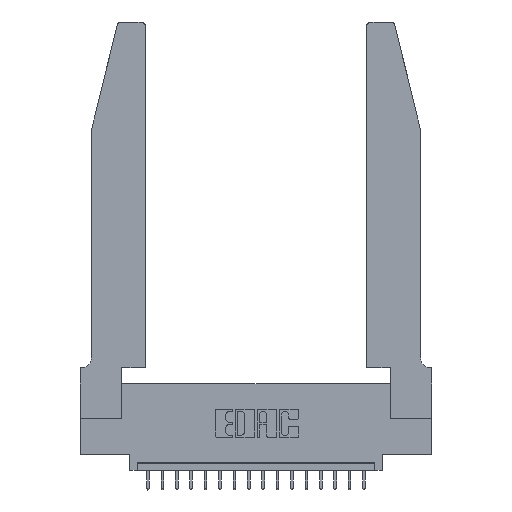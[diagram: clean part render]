
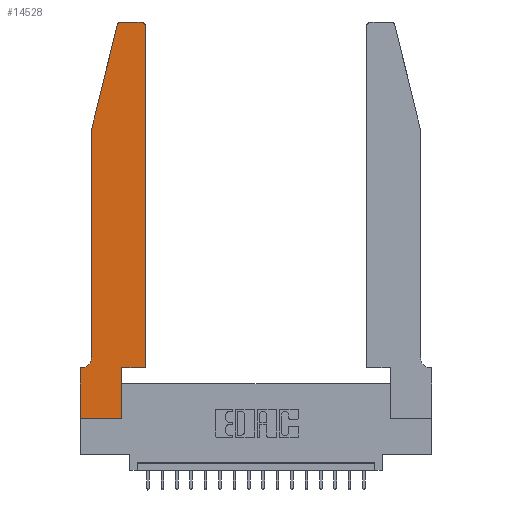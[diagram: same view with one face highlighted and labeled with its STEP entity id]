
A CAD part, top view. The second image highlights one B-rep face of the part: STEP entity #14528.
In plain terms, the highlighted planar face has unit normal (0, 0, 1).
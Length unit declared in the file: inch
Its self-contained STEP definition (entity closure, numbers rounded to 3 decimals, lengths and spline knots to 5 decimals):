
#113 = EDGE_CURVE ( 'NONE', #17525, #18506, #5357, .T. ) ;
#383 = ORIENTED_EDGE ( 'NONE', *, *, #16500, .T. ) ;
#471 = EDGE_CURVE ( 'NONE', #15556, #16411, #1526, .T. ) ;
#630 = EDGE_CURVE ( 'NONE', #4842, #12230, #3383, .T. ) ;
#657 = DIRECTION ( 'NONE',  ( -1., 0., 0. ) ) ;
#890 = DIRECTION ( 'NONE',  ( 0., 0., 1. ) ) ;
#1232 = EDGE_CURVE ( 'NONE', #18089, #17525, #7980, .T. ) ;
#1477 = CARTESIAN_POINT ( 'NONE',  ( 0.284, 2.72, 0.37 ) ) ;
#1526 = LINE ( 'NONE', #9771, #6696 ) ;
#1715 = VECTOR ( 'NONE', #12701, 39.37008 ) ;
#1752 = ORIENTED_EDGE ( 'NONE', *, *, #630, .T. ) ;
#1759 = DIRECTION ( 'NONE',  ( 0., 1., 0. ) ) ;
#1948 = EDGE_CURVE ( 'NONE', #8336, #18089, #7968, .T. ) ;
#2244 = CARTESIAN_POINT ( 'NONE',  ( 0.2865, 0., 0.37 ) ) ;
#2387 = AXIS2_PLACEMENT_3D ( 'NONE', #1477, #890, #7243 ) ;
#2462 = DIRECTION ( 'NONE',  ( 0., -1., 0. ) ) ;
#3156 = VECTOR ( 'NONE', #1759, 39.37008 ) ;
#3383 = CIRCLE ( 'NONE', #2387, 0.03 ) ;
#3620 = ORIENTED_EDGE ( 'NONE', *, *, #471, .T. ) ;
#4023 = VECTOR ( 'NONE', #15811, 39.37008 ) ;
#4216 = ORIENTED_EDGE ( 'NONE', *, *, #17614, .T. ) ;
#4362 = AXIS2_PLACEMENT_3D ( 'NONE', #16031, #18714, #12699 ) ;
#4404 = VERTEX_POINT ( 'NONE', #19523 ) ;
#4630 = DIRECTION ( 'NONE',  ( 1., 0., 0. ) ) ;
#4668 = VECTOR ( 'NONE', #13830, 39.37008 ) ;
#4842 = VERTEX_POINT ( 'NONE', #19663 ) ;
#5047 = CARTESIAN_POINT ( 'NONE',  ( 0.4505, 0.35, 0.37 ) ) ;
#5124 = ORIENTED_EDGE ( 'NONE', *, *, #12304, .T. ) ;
#5357 = CIRCLE ( 'NONE', #4362, 0.03 ) ;
#5645 = ORIENTED_EDGE ( 'NONE', *, *, #17167, .T. ) ;
#5664 = ORIENTED_EDGE ( 'NONE', *, *, #1948, .T. ) ;
#5848 = PLANE ( 'NONE',  #6405 ) ;
#5868 = VERTEX_POINT ( 'NONE', #11637 ) ;
#6051 = CARTESIAN_POINT ( 'NONE',  ( 0.2865, 0.35, 0.37 ) ) ;
#6405 = AXIS2_PLACEMENT_3D ( 'NONE', #20136, #18685, #14142 ) ;
#6568 = DIRECTION ( 'NONE',  ( 0., -1., 0. ) ) ;
#6611 = DIRECTION ( 'NONE',  ( 1., 0., 0. ) ) ;
#6625 = ORIENTED_EDGE ( 'NONE', *, *, #13365, .T. ) ;
#6696 = VECTOR ( 'NONE', #6611, 39.37008 ) ;
#7243 = DIRECTION ( 'NONE',  ( 1., 0., 0. ) ) ;
#7299 = CARTESIAN_POINT ( 'NONE',  ( 0.2605, 2.75, 0.37 ) ) ;
#7926 = CARTESIAN_POINT ( 'NONE',  ( 0.0755, 0.35, 0.37 ) ) ;
#7968 = LINE ( 'NONE', #5047, #11143 ) ;
#7980 = LINE ( 'NONE', #16082, #12696 ) ;
#8004 = CIRCLE ( 'NONE', #11662, 0.07 ) ;
#8146 = LINE ( 'NONE', #19122, #20392 ) ;
#8336 = VERTEX_POINT ( 'NONE', #11892 ) ;
#8852 = VERTEX_POINT ( 'NONE', #17236 ) ;
#9474 = DIRECTION ( 'NONE',  ( 0., 1., 0. ) ) ;
#9771 = CARTESIAN_POINT ( 'NONE',  ( 0., 0., 0.37 ) ) ;
#9949 = EDGE_LOOP ( 'NONE', ( #17696, #1752, #13838, #5645, #5124, #6625, #383, #3620, #4216, #5664, #13246, #10521 ) ) ;
#10457 = LINE ( 'NONE', #7299, #4668 ) ;
#10463 = CARTESIAN_POINT ( 'NONE',  ( 0.4505, 2.72, 0.37 ) ) ;
#10521 = ORIENTED_EDGE ( 'NONE', *, *, #113, .T. ) ;
#11110 = CARTESIAN_POINT ( 'NONE',  ( 0.4505, 0.35, 0.37 ) ) ;
#11143 = VECTOR ( 'NONE', #4630, 39.37008 ) ;
#11169 = EDGE_CURVE ( 'NONE', #18506, #4842, #10457, .T. ) ;
#11637 = CARTESIAN_POINT ( 'NONE',  ( 0.0755, 2., 0.37 ) ) ;
#11662 = AXIS2_PLACEMENT_3D ( 'NONE', #18020, #19658, #657 ) ;
#11877 = CARTESIAN_POINT ( 'NONE',  ( 0.4205, 2.75, 0.37 ) ) ;
#11892 = CARTESIAN_POINT ( 'NONE',  ( 0.2865, 0.35, 0.37 ) ) ;
#12230 = VERTEX_POINT ( 'NONE', #16652 ) ;
#12304 = EDGE_CURVE ( 'NONE', #16963, #4404, #8004, .T. ) ;
#12696 = VECTOR ( 'NONE', #9474, 39.37008 ) ;
#12699 = DIRECTION ( 'NONE',  ( 1., 0., 0. ) ) ;
#12701 = DIRECTION ( 'NONE',  ( -1., 0., 0. ) ) ;
#13188 = LINE ( 'NONE', #7926, #1715 ) ;
#13219 = EDGE_CURVE ( 'NONE', #12230, #5868, #17660, .T. ) ;
#13246 = ORIENTED_EDGE ( 'NONE', *, *, #1232, .T. ) ;
#13361 = CARTESIAN_POINT ( 'NONE',  ( 0.0755, 0.42, 0.37 ) ) ;
#13365 = EDGE_CURVE ( 'NONE', #4404, #8852, #13188, .T. ) ;
#13830 = DIRECTION ( 'NONE',  ( -1., 0., 0. ) ) ;
#13838 = ORIENTED_EDGE ( 'NONE', *, *, #13219, .T. ) ;
#14050 = LINE ( 'NONE', #6051, #3156 ) ;
#14142 = DIRECTION ( 'NONE',  ( 1., 0., 0. ) ) ;
#14528 = ADVANCED_FACE ( 'NONE', ( #18884 ), #5848, .T. ) ;
#15556 = VERTEX_POINT ( 'NONE', #17891 ) ;
#15811 = DIRECTION ( 'NONE',  ( -0.239, -0.971, 0. ) ) ;
#16031 = CARTESIAN_POINT ( 'NONE',  ( 0.4205, 2.72, 0.37 ) ) ;
#16082 = CARTESIAN_POINT ( 'NONE',  ( 0.4505, 0.35, 0.37 ) ) ;
#16411 = VERTEX_POINT ( 'NONE', #2244 ) ;
#16500 = EDGE_CURVE ( 'NONE', #8852, #15556, #16706, .T. ) ;
#16652 = CARTESIAN_POINT ( 'NONE',  ( 0.25487, 2.72718, 0.37 ) ) ;
#16706 = LINE ( 'NONE', #18037, #19354 ) ;
#16963 = VERTEX_POINT ( 'NONE', #13361 ) ;
#17167 = EDGE_CURVE ( 'NONE', #5868, #16963, #8146, .T. ) ;
#17236 = CARTESIAN_POINT ( 'NONE',  ( 0., 0.35, 0.37 ) ) ;
#17260 = CARTESIAN_POINT ( 'NONE',  ( 0.0755, 2., 0.37 ) ) ;
#17525 = VERTEX_POINT ( 'NONE', #10463 ) ;
#17614 = EDGE_CURVE ( 'NONE', #16411, #8336, #14050, .T. ) ;
#17660 = LINE ( 'NONE', #17260, #4023 ) ;
#17696 = ORIENTED_EDGE ( 'NONE', *, *, #11169, .T. ) ;
#17891 = CARTESIAN_POINT ( 'NONE',  ( 0., 0., 0.37 ) ) ;
#18020 = CARTESIAN_POINT ( 'NONE',  ( 0.0055, 0.42, 0.37 ) ) ;
#18037 = CARTESIAN_POINT ( 'NONE',  ( 0., 0., 0.37 ) ) ;
#18089 = VERTEX_POINT ( 'NONE', #11110 ) ;
#18506 = VERTEX_POINT ( 'NONE', #11877 ) ;
#18685 = DIRECTION ( 'NONE',  ( 0., 0., 1. ) ) ;
#18714 = DIRECTION ( 'NONE',  ( 0., 0., 1. ) ) ;
#18884 = FACE_OUTER_BOUND ( 'NONE', #9949, .T. ) ;
#19122 = CARTESIAN_POINT ( 'NONE',  ( 0.0755, 2., 0.37 ) ) ;
#19354 = VECTOR ( 'NONE', #2462, 39.37008 ) ;
#19523 = CARTESIAN_POINT ( 'NONE',  ( 0.0055, 0.35, 0.37 ) ) ;
#19658 = DIRECTION ( 'NONE',  ( 0., 0., -1. ) ) ;
#19663 = CARTESIAN_POINT ( 'NONE',  ( 0.284, 2.75, 0.37 ) ) ;
#20136 = CARTESIAN_POINT ( 'NONE',  ( 0., 0.35, 0.37 ) ) ;
#20392 = VECTOR ( 'NONE', #6568, 39.37008 ) ;
